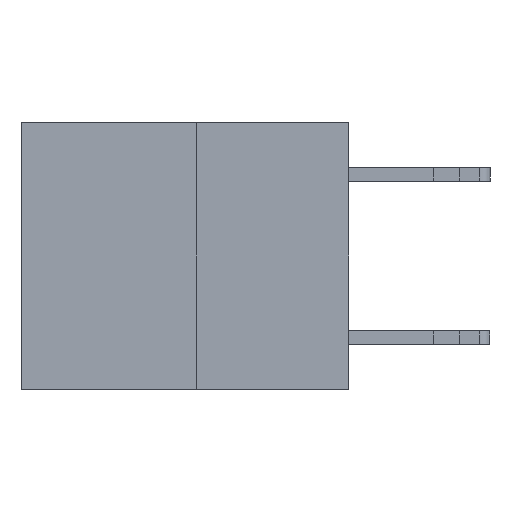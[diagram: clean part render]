
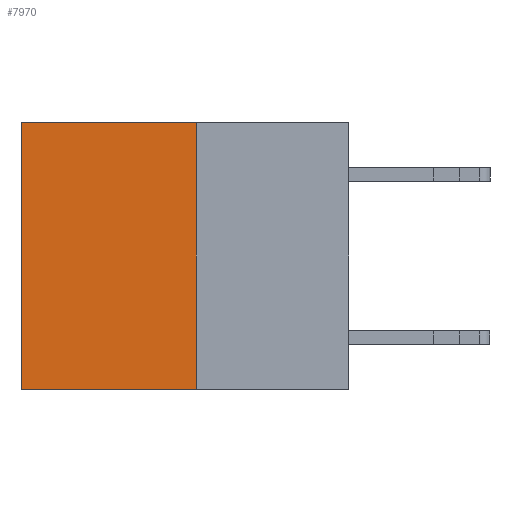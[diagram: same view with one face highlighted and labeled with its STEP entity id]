
A CAD part, left-side view. The second image highlights one B-rep face of the part: STEP entity #7970.
In plain terms, the highlighted planar face has unit normal (-1, 0, 0).
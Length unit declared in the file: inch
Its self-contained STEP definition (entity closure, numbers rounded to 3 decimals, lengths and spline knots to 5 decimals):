
#266 = VECTOR ( 'NONE', #16192, 39.37008 ) ;
#401 = VERTEX_POINT ( 'NONE', #717 ) ;
#454 = FACE_OUTER_BOUND ( 'NONE', #3138, .T. ) ;
#717 = CARTESIAN_POINT ( 'NONE',  ( 0.3165, 0.28, 0. ) ) ;
#1792 = VECTOR ( 'NONE', #15838, 39.37008 ) ;
#2702 = CARTESIAN_POINT ( 'NONE',  ( 0.3165, 0.6, -0.49 ) ) ;
#2971 = CARTESIAN_POINT ( 'NONE',  ( 0.3165, 0.28, -0.49 ) ) ;
#3138 = EDGE_LOOP ( 'NONE', ( #11483, #8105, #12169, #12315 ) ) ;
#3447 = PLANE ( 'NONE',  #13172 ) ;
#3470 = VERTEX_POINT ( 'NONE', #8427 ) ;
#5428 = VERTEX_POINT ( 'NONE', #15835 ) ;
#7426 = LINE ( 'NONE', #9191, #15860 ) ;
#7566 = LINE ( 'NONE', #9799, #266 ) ;
#7925 = EDGE_CURVE ( 'NONE', #3470, #12360, #7566, .T. ) ;
#7970 = ADVANCED_FACE ( 'NONE', ( #454 ), #3447, .F. ) ;
#8105 = ORIENTED_EDGE ( 'NONE', *, *, #11490, .F. ) ;
#8427 = CARTESIAN_POINT ( 'NONE',  ( 0.3165, 0.6, 0. ) ) ;
#9063 = CARTESIAN_POINT ( 'NONE',  ( 0.3165, 0.28, -0.49 ) ) ;
#9191 = CARTESIAN_POINT ( 'NONE',  ( 0.3165, 0.28, 0. ) ) ;
#9799 = CARTESIAN_POINT ( 'NONE',  ( 0.3165, 0.6, -0.49 ) ) ;
#10518 = DIRECTION ( 'NONE',  ( 0., 1., 0. ) ) ;
#11209 = CARTESIAN_POINT ( 'NONE',  ( 0.3165, 0.28, -0.49 ) ) ;
#11483 = ORIENTED_EDGE ( 'NONE', *, *, #7925, .T. ) ;
#11490 = EDGE_CURVE ( 'NONE', #5428, #12360, #14467, .T. ) ;
#12169 = ORIENTED_EDGE ( 'NONE', *, *, #14879, .F. ) ;
#12315 = ORIENTED_EDGE ( 'NONE', *, *, #16017, .T. ) ;
#12360 = VERTEX_POINT ( 'NONE', #2702 ) ;
#12494 = DIRECTION ( 'NONE',  ( 1., 0., 0. ) ) ;
#12887 = LINE ( 'NONE', #9063, #1792 ) ;
#13172 = AXIS2_PLACEMENT_3D ( 'NONE', #11209, #12494, #13788 ) ;
#13788 = DIRECTION ( 'NONE',  ( 0., 0., -1. ) ) ;
#14467 = LINE ( 'NONE', #2971, #15085 ) ;
#14879 = EDGE_CURVE ( 'NONE', #401, #5428, #12887, .T. ) ;
#15085 = VECTOR ( 'NONE', #16276, 39.37008 ) ;
#15835 = CARTESIAN_POINT ( 'NONE',  ( 0.3165, 0.28, -0.49 ) ) ;
#15838 = DIRECTION ( 'NONE',  ( 0., 0., -1. ) ) ;
#15860 = VECTOR ( 'NONE', #10518, 39.37008 ) ;
#16017 = EDGE_CURVE ( 'NONE', #401, #3470, #7426, .T. ) ;
#16192 = DIRECTION ( 'NONE',  ( 0., 0., -1. ) ) ;
#16276 = DIRECTION ( 'NONE',  ( 0., 1., 0. ) ) ;
